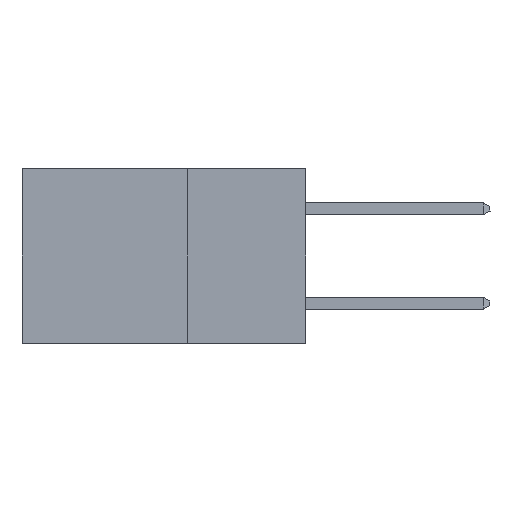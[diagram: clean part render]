
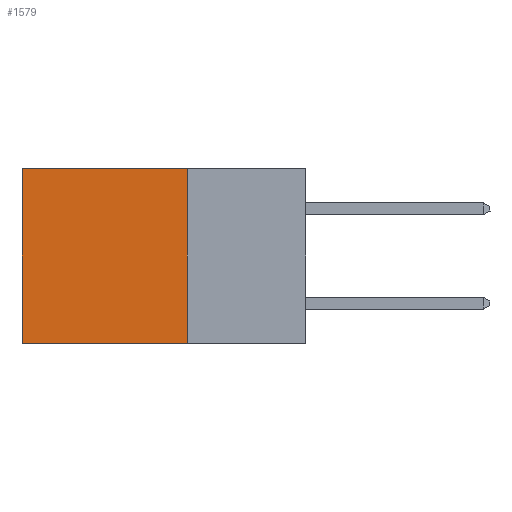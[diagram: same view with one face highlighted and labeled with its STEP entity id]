
A CAD part, left-side view. The second image highlights one B-rep face of the part: STEP entity #1579.
In plain terms, the highlighted planar face has unit normal (-1, 0, 0).
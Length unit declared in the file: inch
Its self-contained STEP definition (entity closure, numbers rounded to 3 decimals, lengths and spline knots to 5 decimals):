
#101 = EDGE_CURVE ( 'NONE', #14087, #2353, #13978, .T. ) ;
#329 = CARTESIAN_POINT ( 'NONE',  ( 0.298, 0.25, -0.37 ) ) ;
#484 = ORIENTED_EDGE ( 'NONE', *, *, #8686, .F. ) ;
#611 = LINE ( 'NONE', #4038, #4889 ) ;
#1423 = LINE ( 'NONE', #13177, #11485 ) ;
#1579 = ADVANCED_FACE ( 'NONE', ( #4614 ), #4759, .F. ) ;
#1592 = EDGE_LOOP ( 'NONE', ( #16183, #7876, #484, #3982 ) ) ;
#2229 = AXIS2_PLACEMENT_3D ( 'NONE', #14956, #8976, #12616 ) ;
#2353 = VERTEX_POINT ( 'NONE', #12688 ) ;
#3144 = LINE ( 'NONE', #7954, #15166 ) ;
#3238 = DIRECTION ( 'NONE',  ( 0., 1., 0. ) ) ;
#3982 = ORIENTED_EDGE ( 'NONE', *, *, #101, .T. ) ;
#4038 = CARTESIAN_POINT ( 'NONE',  ( 0.298, 0.25, -0.37 ) ) ;
#4614 = FACE_OUTER_BOUND ( 'NONE', #1592, .T. ) ;
#4759 = PLANE ( 'NONE',  #2229 ) ;
#4889 = VECTOR ( 'NONE', #9158, 39.37008 ) ;
#5530 = DIRECTION ( 'NONE',  ( 0., 0., -1. ) ) ;
#6782 = EDGE_CURVE ( 'NONE', #2353, #8820, #1423, .T. ) ;
#7230 = DIRECTION ( 'NONE',  ( 0., 0., -1. ) ) ;
#7681 = EDGE_CURVE ( 'NONE', #7684, #8820, #611, .T. ) ;
#7684 = VERTEX_POINT ( 'NONE', #329 ) ;
#7876 = ORIENTED_EDGE ( 'NONE', *, *, #7681, .F. ) ;
#7954 = CARTESIAN_POINT ( 'NONE',  ( 0.298, 0.25, 0. ) ) ;
#8686 = EDGE_CURVE ( 'NONE', #14087, #7684, #3144, .T. ) ;
#8820 = VERTEX_POINT ( 'NONE', #12000 ) ;
#8976 = DIRECTION ( 'NONE',  ( 1., 0., 0. ) ) ;
#9158 = DIRECTION ( 'NONE',  ( 0., 1., 0. ) ) ;
#9525 = CARTESIAN_POINT ( 'NONE',  ( 0.298, 0.25, 0. ) ) ;
#10220 = CARTESIAN_POINT ( 'NONE',  ( 0.298, 0.25, 0. ) ) ;
#11485 = VECTOR ( 'NONE', #7230, 39.37008 ) ;
#11996 = VECTOR ( 'NONE', #3238, 39.37008 ) ;
#12000 = CARTESIAN_POINT ( 'NONE',  ( 0.298, 0.6, -0.37 ) ) ;
#12616 = DIRECTION ( 'NONE',  ( 0., 0., -1. ) ) ;
#12688 = CARTESIAN_POINT ( 'NONE',  ( 0.298, 0.6, 0. ) ) ;
#13177 = CARTESIAN_POINT ( 'NONE',  ( 0.298, 0.6, 0. ) ) ;
#13978 = LINE ( 'NONE', #9525, #11996 ) ;
#14087 = VERTEX_POINT ( 'NONE', #10220 ) ;
#14956 = CARTESIAN_POINT ( 'NONE',  ( 0.298, 0.25, 0. ) ) ;
#15166 = VECTOR ( 'NONE', #5530, 39.37008 ) ;
#16183 = ORIENTED_EDGE ( 'NONE', *, *, #6782, .T. ) ;
